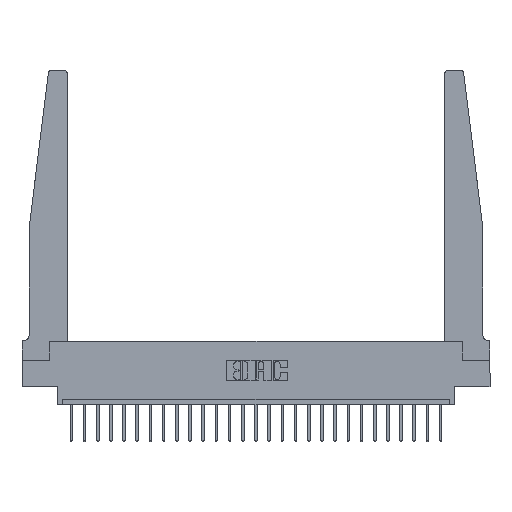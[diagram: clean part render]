
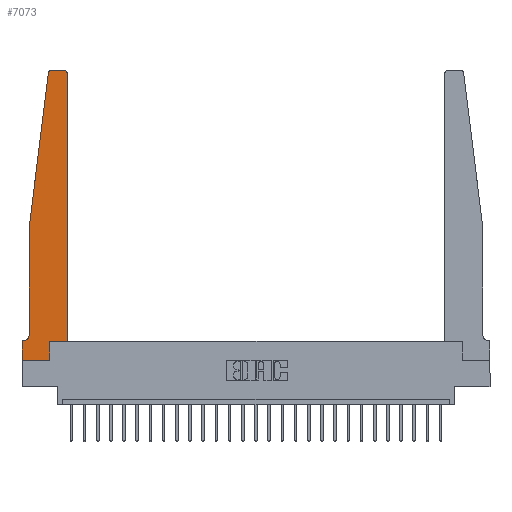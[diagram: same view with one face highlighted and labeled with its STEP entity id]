
A CAD part, top view. The second image highlights one B-rep face of the part: STEP entity #7073.
In plain terms, the highlighted planar face has unit normal (0, 0, 1).
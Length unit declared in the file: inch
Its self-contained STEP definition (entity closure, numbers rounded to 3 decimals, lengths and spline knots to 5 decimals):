
#148 = VECTOR ( 'NONE', #19646, 39.37008 ) ;
#946 = DIRECTION ( 'NONE',  ( 0., 0., 1. ) ) ;
#1467 = VECTOR ( 'NONE', #7288, 39.37008 ) ;
#1829 = ORIENTED_EDGE ( 'NONE', *, *, #23759, .T. ) ;
#1910 = ORIENTED_EDGE ( 'NONE', *, *, #8652, .T. ) ;
#1961 = CARTESIAN_POINT ( 'NONE',  ( 0.425, 0.18, 0.37 ) ) ;
#2011 = DIRECTION ( 'NONE',  ( 1., 0., 0. ) ) ;
#2310 = EDGE_CURVE ( 'NONE', #17970, #5143, #16241, .T. ) ;
#2450 = EDGE_CURVE ( 'NONE', #22601, #4936, #21001, .T. ) ;
#2499 = VERTEX_POINT ( 'NONE', #17565 ) ;
#2988 = DIRECTION ( 'NONE',  ( 1., 0., 0. ) ) ;
#3313 = CARTESIAN_POINT ( 'NONE',  ( 0.065, 1.25, 0.37 ) ) ;
#3580 = CARTESIAN_POINT ( 'NONE',  ( 0.2605, 0., 0.37 ) ) ;
#3704 = CARTESIAN_POINT ( 'NONE',  ( 0., 0., 0.37 ) ) ;
#3906 = LINE ( 'NONE', #12411, #148 ) ;
#3928 = ORIENTED_EDGE ( 'NONE', *, *, #19479, .T. ) ;
#4180 = CARTESIAN_POINT ( 'NONE',  ( 0., 0., 0.37 ) ) ;
#4276 = DIRECTION ( 'NONE',  ( 0., 0., -1. ) ) ;
#4331 = VECTOR ( 'NONE', #23800, 39.37008 ) ;
#4361 = CARTESIAN_POINT ( 'NONE',  ( 0.2605, 0.18, 0.37 ) ) ;
#4511 = LINE ( 'NONE', #4640, #14294 ) ;
#4640 = CARTESIAN_POINT ( 'NONE',  ( 0., 0., 0.37 ) ) ;
#4790 = CARTESIAN_POINT ( 'NONE',  ( 0.065, 1.25, 0.37 ) ) ;
#4823 = VERTEX_POINT ( 'NONE', #4790 ) ;
#4936 = VERTEX_POINT ( 'NONE', #22420 ) ;
#5143 = VERTEX_POINT ( 'NONE', #1961 ) ;
#5327 = ORIENTED_EDGE ( 'NONE', *, *, #17696, .T. ) ;
#5421 = AXIS2_PLACEMENT_3D ( 'NONE', #14559, #4276, #23851 ) ;
#5542 = VERTEX_POINT ( 'NONE', #3704 ) ;
#6007 = EDGE_CURVE ( 'NONE', #5542, #24410, #4511, .T. ) ;
#6078 = LINE ( 'NONE', #4180, #11963 ) ;
#6116 = LINE ( 'NONE', #4361, #4331 ) ;
#6708 = DIRECTION ( 'NONE',  ( 1., 0., 0. ) ) ;
#6769 = AXIS2_PLACEMENT_3D ( 'NONE', #12145, #946, #24213 ) ;
#7073 = ADVANCED_FACE ( 'NONE', ( #24460 ), #14435, .T. ) ;
#7288 = DIRECTION ( 'NONE',  ( 0., 1., 0. ) ) ;
#7485 = VECTOR ( 'NONE', #7660, 39.37008 ) ;
#7660 = DIRECTION ( 'NONE',  ( -1., 0., 0. ) ) ;
#8314 = EDGE_CURVE ( 'NONE', #16252, #5542, #6078, .T. ) ;
#8652 = EDGE_CURVE ( 'NONE', #4823, #13671, #3906, .T. ) ;
#8683 = DIRECTION ( 'NONE',  ( -0.122, -0.992, 0. ) ) ;
#9285 = CARTESIAN_POINT ( 'NONE',  ( 0.425, 2.72, 0.37 ) ) ;
#10501 = CARTESIAN_POINT ( 'NONE',  ( 0.395, 2.75, 0.37 ) ) ;
#11109 = DIRECTION ( 'NONE',  ( -1., 0., 0. ) ) ;
#11373 = ORIENTED_EDGE ( 'NONE', *, *, #23145, .T. ) ;
#11377 = ORIENTED_EDGE ( 'NONE', *, *, #8314, .T. ) ;
#11517 = AXIS2_PLACEMENT_3D ( 'NONE', #18245, #23964, #20519 ) ;
#11536 = EDGE_CURVE ( 'NONE', #2499, #16252, #13623, .T. ) ;
#11787 = CARTESIAN_POINT ( 'NONE',  ( 0.065, 0.2375, 0.37 ) ) ;
#11963 = VECTOR ( 'NONE', #19677, 39.37008 ) ;
#12136 = CARTESIAN_POINT ( 'NONE',  ( 0.24675, 2.72367, 0.37 ) ) ;
#12145 = CARTESIAN_POINT ( 'NONE',  ( 0.395, 2.72, 0.37 ) ) ;
#12311 = VECTOR ( 'NONE', #8683, 39.37008 ) ;
#12333 = CARTESIAN_POINT ( 'NONE',  ( 0., 0.1875, 0.37 ) ) ;
#12411 = CARTESIAN_POINT ( 'NONE',  ( 0.065, 1.25, 0.37 ) ) ;
#12617 = CARTESIAN_POINT ( 'NONE',  ( 0.2605, 0.18, 0.37 ) ) ;
#13136 = CIRCLE ( 'NONE', #5421, 0.05 ) ;
#13223 = CIRCLE ( 'NONE', #21742, 0.03 ) ;
#13623 = LINE ( 'NONE', #15902, #7485 ) ;
#13671 = VERTEX_POINT ( 'NONE', #11787 ) ;
#14248 = ORIENTED_EDGE ( 'NONE', *, *, #2310, .T. ) ;
#14294 = VECTOR ( 'NONE', #2988, 39.37008 ) ;
#14435 = PLANE ( 'NONE',  #11517 ) ;
#14559 = CARTESIAN_POINT ( 'NONE',  ( 0.015, 0.2375, 0.37 ) ) ;
#14625 = ORIENTED_EDGE ( 'NONE', *, *, #6007, .T. ) ;
#14910 = CARTESIAN_POINT ( 'NONE',  ( 0.425, 0.18, 0.37 ) ) ;
#15037 = CARTESIAN_POINT ( 'NONE',  ( 0.25, 2.75, 0.37 ) ) ;
#15280 = LINE ( 'NONE', #14910, #1467 ) ;
#15902 = CARTESIAN_POINT ( 'NONE',  ( 0.065, 0.1875, 0.37 ) ) ;
#15989 = CARTESIAN_POINT ( 'NONE',  ( 0.27653, 2.72, 0.37 ) ) ;
#16241 = LINE ( 'NONE', #18390, #16868 ) ;
#16252 = VERTEX_POINT ( 'NONE', #12333 ) ;
#16582 = EDGE_LOOP ( 'NONE', ( #18571, #5327, #11373, #1910, #1829, #19530, #11377, #14625, #3928, #14248, #21614, #17763 ) ) ;
#16868 = VECTOR ( 'NONE', #6708, 39.37008 ) ;
#16985 = VERTEX_POINT ( 'NONE', #12136 ) ;
#17247 = EDGE_CURVE ( 'NONE', #5143, #24748, #15280, .T. ) ;
#17565 = CARTESIAN_POINT ( 'NONE',  ( 0.015, 0.1875, 0.37 ) ) ;
#17696 = EDGE_CURVE ( 'NONE', #4936, #16985, #13223, .T. ) ;
#17763 = ORIENTED_EDGE ( 'NONE', *, *, #20389, .T. ) ;
#17970 = VERTEX_POINT ( 'NONE', #12617 ) ;
#18245 = CARTESIAN_POINT ( 'NONE',  ( 0., 0.1875, 0.37 ) ) ;
#18390 = CARTESIAN_POINT ( 'NONE',  ( 0.425, 0.18, 0.37 ) ) ;
#18571 = ORIENTED_EDGE ( 'NONE', *, *, #2450, .T. ) ;
#19479 = EDGE_CURVE ( 'NONE', #24410, #17970, #6116, .T. ) ;
#19530 = ORIENTED_EDGE ( 'NONE', *, *, #11536, .T. ) ;
#19646 = DIRECTION ( 'NONE',  ( 0., -1., 0. ) ) ;
#19677 = DIRECTION ( 'NONE',  ( 0., -1., 0. ) ) ;
#20153 = CIRCLE ( 'NONE', #6769, 0.03 ) ;
#20328 = VECTOR ( 'NONE', #11109, 39.37008 ) ;
#20389 = EDGE_CURVE ( 'NONE', #24748, #22601, #20153, .T. ) ;
#20519 = DIRECTION ( 'NONE',  ( 1., 0., 0. ) ) ;
#21001 = LINE ( 'NONE', #15037, #20328 ) ;
#21614 = ORIENTED_EDGE ( 'NONE', *, *, #17247, .T. ) ;
#21694 = DIRECTION ( 'NONE',  ( 0., 0., 1. ) ) ;
#21742 = AXIS2_PLACEMENT_3D ( 'NONE', #15989, #21694, #2011 ) ;
#22420 = CARTESIAN_POINT ( 'NONE',  ( 0.27653, 2.75, 0.37 ) ) ;
#22503 = LINE ( 'NONE', #3313, #12311 ) ;
#22601 = VERTEX_POINT ( 'NONE', #10501 ) ;
#23145 = EDGE_CURVE ( 'NONE', #16985, #4823, #22503, .T. ) ;
#23759 = EDGE_CURVE ( 'NONE', #13671, #2499, #13136, .T. ) ;
#23800 = DIRECTION ( 'NONE',  ( 0., 1., 0. ) ) ;
#23851 = DIRECTION ( 'NONE',  ( -1., 0., 0. ) ) ;
#23964 = DIRECTION ( 'NONE',  ( 0., 0., 1. ) ) ;
#24213 = DIRECTION ( 'NONE',  ( 1., 0., 0. ) ) ;
#24410 = VERTEX_POINT ( 'NONE', #3580 ) ;
#24460 = FACE_OUTER_BOUND ( 'NONE', #16582, .T. ) ;
#24748 = VERTEX_POINT ( 'NONE', #9285 ) ;
